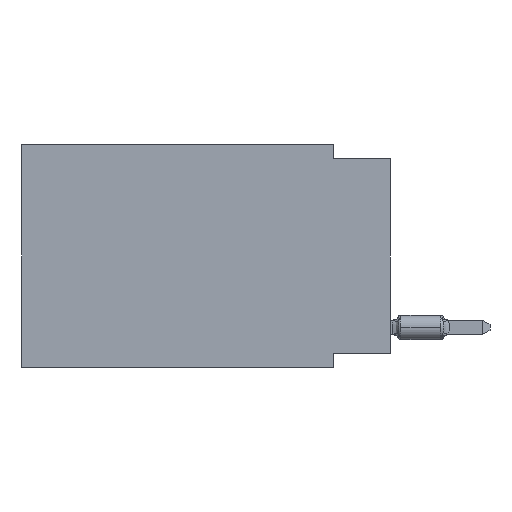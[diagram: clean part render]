
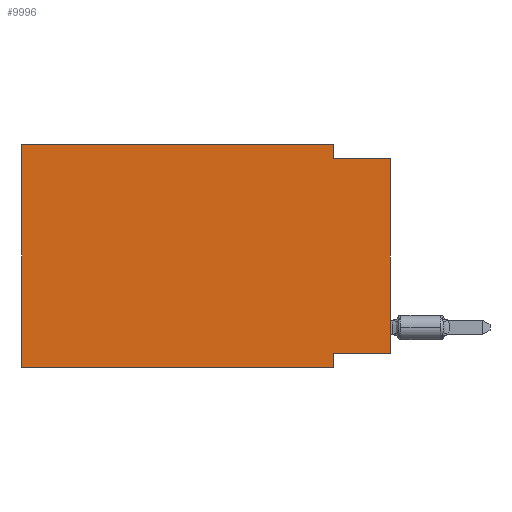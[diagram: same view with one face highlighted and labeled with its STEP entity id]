
A CAD part, left-side view. The second image highlights one B-rep face of the part: STEP entity #9996.
In plain terms, the highlighted planar face has unit normal (-1, 0, 0).
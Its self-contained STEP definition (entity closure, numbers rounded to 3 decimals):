
#195 = DIRECTION ( 'NONE',  ( 1., 0., 0. ) ) ;
#666 = CARTESIAN_POINT ( 'NONE',  ( 0., 2.54, -9.906 ) ) ;
#1513 = CARTESIAN_POINT ( 'NONE',  ( 0., 16.383, 0. ) ) ;
#1536 = CARTESIAN_POINT ( 'NONE',  ( 0., 16.383, -9.906 ) ) ;
#1769 = CARTESIAN_POINT ( 'NONE',  ( 0., 0., 0. ) ) ;
#1934 = LINE ( 'NONE', #9226, #20064 ) ;
#1994 = DIRECTION ( 'NONE',  ( 0., 0., 1. ) ) ;
#2113 = CARTESIAN_POINT ( 'NONE',  ( 0., 2.54, -0.635 ) ) ;
#2169 = DIRECTION ( 'NONE',  ( 0., 0., -1. ) ) ;
#2598 = DIRECTION ( 'NONE',  ( 0., 0., -1. ) ) ;
#3046 = CARTESIAN_POINT ( 'NONE',  ( 0., 0., -0.635 ) ) ;
#3057 = VERTEX_POINT ( 'NONE', #4914 ) ;
#3745 = EDGE_CURVE ( 'NONE', #7139, #3057, #22366, .T. ) ;
#3874 = DIRECTION ( 'NONE',  ( 0., 1., 0. ) ) ;
#4594 = LINE ( 'NONE', #3046, #12192 ) ;
#4914 = CARTESIAN_POINT ( 'NONE',  ( 0., 2.54, -9.271 ) ) ;
#5062 = VECTOR ( 'NONE', #2598, 1000. ) ;
#5159 = EDGE_CURVE ( 'NONE', #16969, #14046, #4594, .T. ) ;
#5376 = LINE ( 'NONE', #666, #5062 ) ;
#6987 = DIRECTION ( 'NONE',  ( 0., -1., 0. ) ) ;
#7139 = VERTEX_POINT ( 'NONE', #8466 ) ;
#7278 = CARTESIAN_POINT ( 'NONE',  ( 0., 2.54, 0. ) ) ;
#7508 = DIRECTION ( 'NONE',  ( 0., 0., -1. ) ) ;
#8161 = ORIENTED_EDGE ( 'NONE', *, *, #3745, .F. ) ;
#8466 = CARTESIAN_POINT ( 'NONE',  ( 0., 0., -9.271 ) ) ;
#8576 = ORIENTED_EDGE ( 'NONE', *, *, #5159, .F. ) ;
#9226 = CARTESIAN_POINT ( 'NONE',  ( 0., 2.54, 0. ) ) ;
#9293 = LINE ( 'NONE', #1769, #20975 ) ;
#9729 = EDGE_CURVE ( 'NONE', #17464, #9993, #11385, .T. ) ;
#9993 = VERTEX_POINT ( 'NONE', #7278 ) ;
#9996 = ADVANCED_FACE ( 'NONE', ( #20261 ), #20493, .F. ) ;
#10175 = EDGE_CURVE ( 'NONE', #19996, #17464, #23117, .T. ) ;
#10341 = DIRECTION ( 'NONE',  ( 0., -1., 0. ) ) ;
#11242 = VECTOR ( 'NONE', #6987, 1000. ) ;
#11385 = LINE ( 'NONE', #13184, #11242 ) ;
#12192 = VECTOR ( 'NONE', #10341, 1000. ) ;
#12227 = DIRECTION ( 'NONE',  ( 0., -1., 0. ) ) ;
#12430 = CARTESIAN_POINT ( 'NONE',  ( 0., 0., -0.635 ) ) ;
#13184 = CARTESIAN_POINT ( 'NONE',  ( 0., 16.383, 0. ) ) ;
#14046 = VERTEX_POINT ( 'NONE', #12430 ) ;
#14071 = ORIENTED_EDGE ( 'NONE', *, *, #10175, .F. ) ;
#14079 = ORIENTED_EDGE ( 'NONE', *, *, #15421, .F. ) ;
#14413 = AXIS2_PLACEMENT_3D ( 'NONE', #16638, #195, #7508 ) ;
#14960 = EDGE_CURVE ( 'NONE', #9993, #16969, #1934, .T. ) ;
#15287 = EDGE_CURVE ( 'NONE', #19996, #22351, #16184, .T. ) ;
#15421 = EDGE_CURVE ( 'NONE', #3057, #22351, #5376, .T. ) ;
#15489 = CARTESIAN_POINT ( 'NONE',  ( 0., 16.383, 0. ) ) ;
#15681 = DIRECTION ( 'NONE',  ( 0., 0., 1. ) ) ;
#15946 = VECTOR ( 'NONE', #15681, 1000. ) ;
#16184 = LINE ( 'NONE', #23160, #20784 ) ;
#16348 = ORIENTED_EDGE ( 'NONE', *, *, #18886, .T. ) ;
#16638 = CARTESIAN_POINT ( 'NONE',  ( 0., 16.383, 0. ) ) ;
#16969 = VERTEX_POINT ( 'NONE', #2113 ) ;
#17022 = ORIENTED_EDGE ( 'NONE', *, *, #15287, .T. ) ;
#17154 = VECTOR ( 'NONE', #3874, 1000. ) ;
#17433 = ORIENTED_EDGE ( 'NONE', *, *, #14960, .F. ) ;
#17464 = VERTEX_POINT ( 'NONE', #15489 ) ;
#18289 = CARTESIAN_POINT ( 'NONE',  ( 0., 2.54, -9.906 ) ) ;
#18886 = EDGE_CURVE ( 'NONE', #7139, #14046, #9293, .T. ) ;
#19996 = VERTEX_POINT ( 'NONE', #1536 ) ;
#20064 = VECTOR ( 'NONE', #2169, 1000. ) ;
#20261 = FACE_OUTER_BOUND ( 'NONE', #21270, .T. ) ;
#20333 = CARTESIAN_POINT ( 'NONE',  ( 0., 0., -9.271 ) ) ;
#20493 = PLANE ( 'NONE',  #14413 ) ;
#20784 = VECTOR ( 'NONE', #12227, 1000. ) ;
#20975 = VECTOR ( 'NONE', #1994, 1000. ) ;
#21270 = EDGE_LOOP ( 'NONE', ( #16348, #8576, #17433, #21811, #14071, #17022, #14079, #8161 ) ) ;
#21811 = ORIENTED_EDGE ( 'NONE', *, *, #9729, .F. ) ;
#22351 = VERTEX_POINT ( 'NONE', #18289 ) ;
#22366 = LINE ( 'NONE', #20333, #17154 ) ;
#23117 = LINE ( 'NONE', #1513, #15946 ) ;
#23160 = CARTESIAN_POINT ( 'NONE',  ( 0., 16.383, -9.906 ) ) ;
